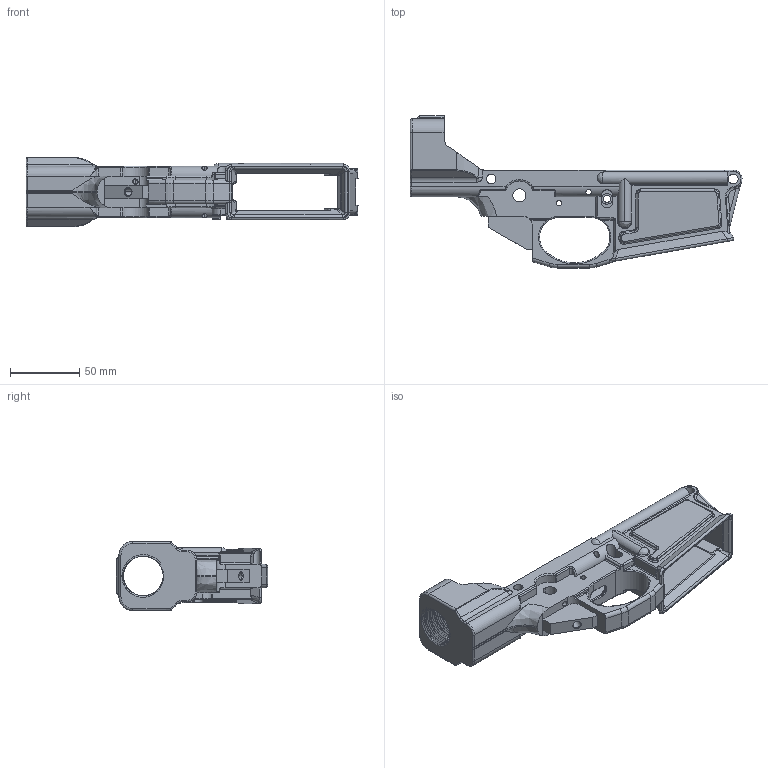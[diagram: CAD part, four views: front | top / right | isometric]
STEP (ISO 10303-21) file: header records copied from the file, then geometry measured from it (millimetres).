
FILE_DESCRIPTION (( 'STEP AP214' ), '1' );
FILE_NAME ('Nephilim_AR-10_V2.STEP', '2015-05-16T20:39:45', ( 'WarFairy' ), ( '' ), 'SwSTEP 2.0', 'SolidWorks 2015', '' );
FILE_SCHEMA (( 'AUTOMOTIVE_DESIGN' ));
Length unit declared in the file: millimetre
Products named in the file (1): Nephilim_AR-10_V2
Bounding box: 239.65 x 109.71 x 50 mm (x, y, z)
Volume: 208567.1 mm3; surface area: 71011.7 mm2
Topology: 1 solids, 1 shells, 640 faces, 1727 edges, 1069 vertices
Faces by surface type: cylinder 308, plane 143, bspline 122, torus 61, sphere 4, cone 2
Entity records: 42948 total; most frequent: CARTESIAN_POINT 22421, ORIENTED_EDGE 3422, DIRECTION 2824, EDGE_CURVE 1711, AXIS2_PLACEMENT_3D 1069, VERTEX_POINT 1069, LINE 686, VECTOR 686
